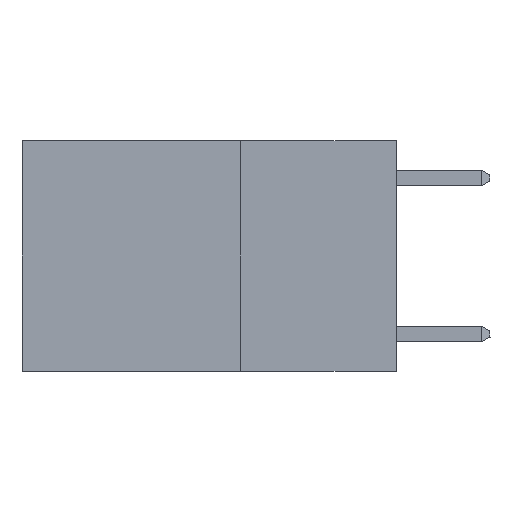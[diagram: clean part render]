
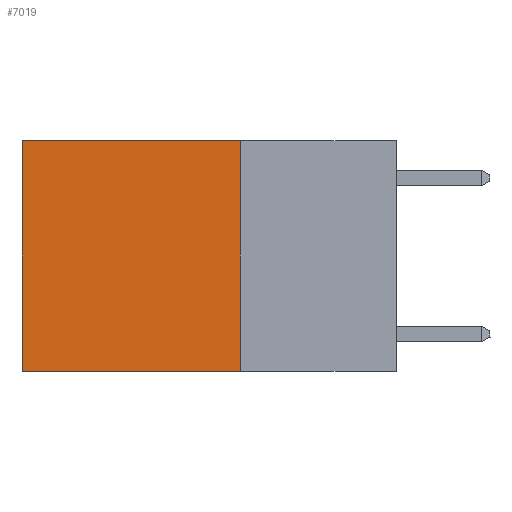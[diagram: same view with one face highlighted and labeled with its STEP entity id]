
A CAD part, left-side view. The second image highlights one B-rep face of the part: STEP entity #7019.
In plain terms, the highlighted planar face has unit normal (-1, 0, 0).
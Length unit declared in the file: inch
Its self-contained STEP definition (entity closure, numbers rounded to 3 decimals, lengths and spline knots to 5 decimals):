
#165 = CARTESIAN_POINT ( 'NONE',  ( 0.2625, 0.6, -0.37 ) ) ;
#208 = LINE ( 'NONE', #3004, #6219 ) ;
#723 = EDGE_CURVE ( 'NONE', #2133, #2771, #3457, .T. ) ;
#794 = LINE ( 'NONE', #1608, #2590 ) ;
#1066 = ORIENTED_EDGE ( 'NONE', *, *, #3049, .T. ) ;
#1082 = CARTESIAN_POINT ( 'NONE',  ( 0.2625, 0.25, -0.37 ) ) ;
#1608 = CARTESIAN_POINT ( 'NONE',  ( 0.2625, 0.25, -0.37 ) ) ;
#2133 = VERTEX_POINT ( 'NONE', #8684 ) ;
#2337 = DIRECTION ( 'NONE',  ( 1., 0., 0. ) ) ;
#2383 = CARTESIAN_POINT ( 'NONE',  ( 0.2625, 0.6, 0. ) ) ;
#2590 = VECTOR ( 'NONE', #6894, 39.37008 ) ;
#2771 = VERTEX_POINT ( 'NONE', #1082 ) ;
#3004 = CARTESIAN_POINT ( 'NONE',  ( 0.2625, 0.25, 0. ) ) ;
#3049 = EDGE_CURVE ( 'NONE', #6464, #6539, #7665, .T. ) ;
#3457 = LINE ( 'NONE', #7488, #5567 ) ;
#3618 = EDGE_LOOP ( 'NONE', ( #1066, #7297, #9142, #8077 ) ) ;
#3769 = DIRECTION ( 'NONE',  ( 0., 0., -1. ) ) ;
#3790 = VECTOR ( 'NONE', #6963, 39.37008 ) ;
#4602 = PLANE ( 'NONE',  #6982 ) ;
#5446 = DIRECTION ( 'NONE',  ( 0., 1., 0. ) ) ;
#5567 = VECTOR ( 'NONE', #3769, 39.37008 ) ;
#6219 = VECTOR ( 'NONE', #5446, 39.37008 ) ;
#6394 = EDGE_CURVE ( 'NONE', #2133, #6464, #208, .T. ) ;
#6464 = VERTEX_POINT ( 'NONE', #2383 ) ;
#6539 = VERTEX_POINT ( 'NONE', #165 ) ;
#6862 = CARTESIAN_POINT ( 'NONE',  ( 0.2625, 0.6, 0. ) ) ;
#6894 = DIRECTION ( 'NONE',  ( 0., 1., 0. ) ) ;
#6963 = DIRECTION ( 'NONE',  ( 0., 0., -1. ) ) ;
#6982 = AXIS2_PLACEMENT_3D ( 'NONE', #8133, #2337, #7541 ) ;
#7019 = ADVANCED_FACE ( 'NONE', ( #8076 ), #4602, .F. ) ;
#7297 = ORIENTED_EDGE ( 'NONE', *, *, #7859, .F. ) ;
#7488 = CARTESIAN_POINT ( 'NONE',  ( 0.2625, 0.25, 0. ) ) ;
#7541 = DIRECTION ( 'NONE',  ( 0., 0., -1. ) ) ;
#7665 = LINE ( 'NONE', #6862, #3790 ) ;
#7859 = EDGE_CURVE ( 'NONE', #2771, #6539, #794, .T. ) ;
#8076 = FACE_OUTER_BOUND ( 'NONE', #3618, .T. ) ;
#8077 = ORIENTED_EDGE ( 'NONE', *, *, #6394, .T. ) ;
#8133 = CARTESIAN_POINT ( 'NONE',  ( 0.2625, 0.25, 0. ) ) ;
#8684 = CARTESIAN_POINT ( 'NONE',  ( 0.2625, 0.25, 0. ) ) ;
#9142 = ORIENTED_EDGE ( 'NONE', *, *, #723, .F. ) ;
